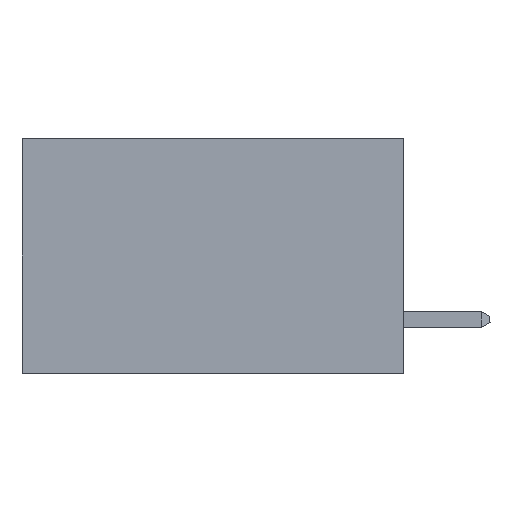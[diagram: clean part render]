
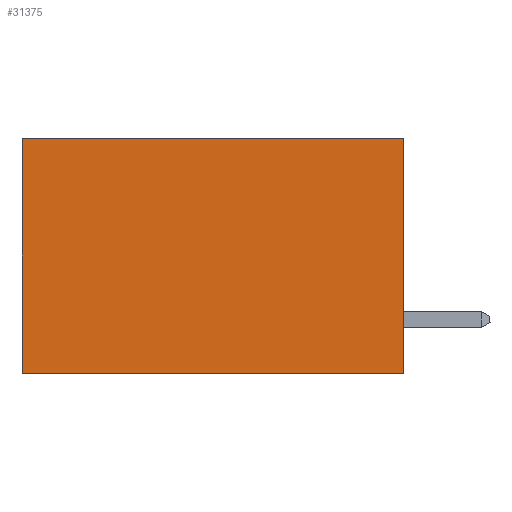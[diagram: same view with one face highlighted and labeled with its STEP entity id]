
A CAD part, left-side view. The second image highlights one B-rep face of the part: STEP entity #31375.
In plain terms, the highlighted planar face has unit normal (-1, 0, 0).
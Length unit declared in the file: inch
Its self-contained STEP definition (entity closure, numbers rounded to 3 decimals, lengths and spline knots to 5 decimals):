
#2127 = EDGE_CURVE ( 'NONE', #34842, #18339, #41924, .T. ) ;
#2922 = AXIS2_PLACEMENT_3D ( 'NONE', #29695, #33425, #10964 ) ;
#3587 = DIRECTION ( 'NONE',  ( 0., 0., -1. ) ) ;
#3712 = DIRECTION ( 'NONE',  ( 0., 1., 0. ) ) ;
#4605 = CARTESIAN_POINT ( 'NONE',  ( 0.2875, 0., 0. ) ) ;
#5154 = LINE ( 'NONE', #18734, #24089 ) ;
#7352 = CARTESIAN_POINT ( 'NONE',  ( 0.2875, 0., -0.37 ) ) ;
#8913 = LINE ( 'NONE', #48597, #45199 ) ;
#10081 = CARTESIAN_POINT ( 'NONE',  ( 0.2875, 0., 0. ) ) ;
#10964 = DIRECTION ( 'NONE',  ( 0., 0., -1. ) ) ;
#11190 = CARTESIAN_POINT ( 'NONE',  ( 0.2875, 0., -0.37 ) ) ;
#15366 = EDGE_LOOP ( 'NONE', ( #25475, #32689, #35028, #45107 ) ) ;
#16771 = EDGE_CURVE ( 'NONE', #48538, #34842, #41242, .T. ) ;
#16916 = FACE_OUTER_BOUND ( 'NONE', #15366, .T. ) ;
#18339 = VERTEX_POINT ( 'NONE', #24969 ) ;
#18734 = CARTESIAN_POINT ( 'NONE',  ( 0.2875, 0.6, 0. ) ) ;
#19667 = EDGE_CURVE ( 'NONE', #48538, #21070, #8913, .T. ) ;
#20969 = EDGE_CURVE ( 'NONE', #21070, #18339, #5154, .T. ) ;
#21070 = VERTEX_POINT ( 'NONE', #26680 ) ;
#24089 = VECTOR ( 'NONE', #3587, 39.37008 ) ;
#24969 = CARTESIAN_POINT ( 'NONE',  ( 0.2875, 0.6, -0.37 ) ) ;
#25475 = ORIENTED_EDGE ( 'NONE', *, *, #20969, .T. ) ;
#25893 = PLANE ( 'NONE',  #2922 ) ;
#26680 = CARTESIAN_POINT ( 'NONE',  ( 0.2875, 0.6, 0. ) ) ;
#29695 = CARTESIAN_POINT ( 'NONE',  ( 0.2875, 0., 0. ) ) ;
#31157 = DIRECTION ( 'NONE',  ( 0., 0., -1. ) ) ;
#31375 = ADVANCED_FACE ( 'NONE', ( #16916 ), #25893, .F. ) ;
#31387 = VECTOR ( 'NONE', #31157, 39.37008 ) ;
#32689 = ORIENTED_EDGE ( 'NONE', *, *, #2127, .F. ) ;
#33254 = VECTOR ( 'NONE', #38512, 39.37008 ) ;
#33425 = DIRECTION ( 'NONE',  ( 1., 0., 0. ) ) ;
#34842 = VERTEX_POINT ( 'NONE', #7352 ) ;
#35028 = ORIENTED_EDGE ( 'NONE', *, *, #16771, .F. ) ;
#38512 = DIRECTION ( 'NONE',  ( 0., 1., 0. ) ) ;
#41242 = LINE ( 'NONE', #4605, #31387 ) ;
#41924 = LINE ( 'NONE', #11190, #33254 ) ;
#45107 = ORIENTED_EDGE ( 'NONE', *, *, #19667, .T. ) ;
#45199 = VECTOR ( 'NONE', #3712, 39.37008 ) ;
#48538 = VERTEX_POINT ( 'NONE', #10081 ) ;
#48597 = CARTESIAN_POINT ( 'NONE',  ( 0.2875, 0., 0. ) ) ;
